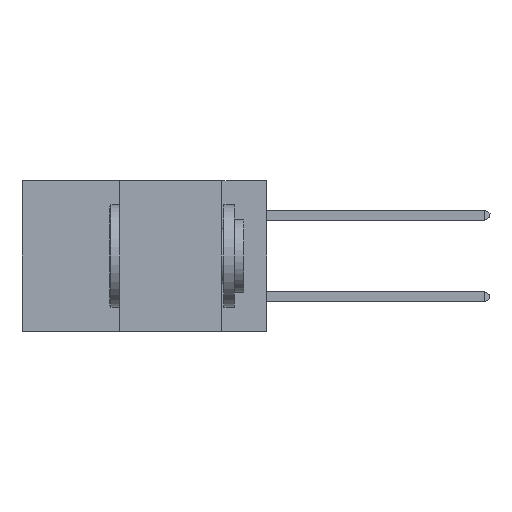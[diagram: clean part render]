
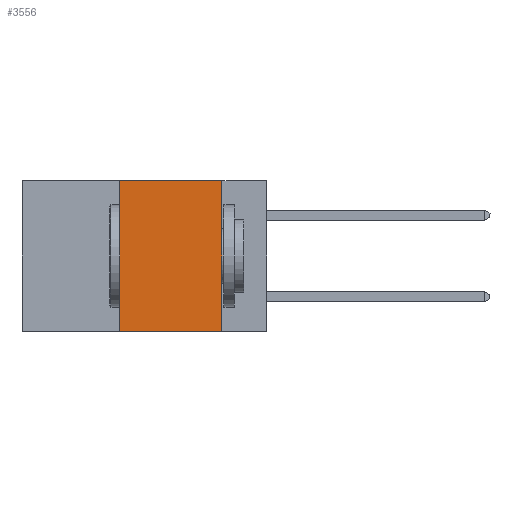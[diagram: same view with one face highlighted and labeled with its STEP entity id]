
A CAD part, left-side view. The second image highlights one B-rep face of the part: STEP entity #3556.
In plain terms, the highlighted planar face has unit normal (-1, 0, 0).
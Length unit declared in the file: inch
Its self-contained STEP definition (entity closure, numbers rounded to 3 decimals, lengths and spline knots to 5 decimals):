
#459 = ORIENTED_EDGE ( 'NONE', *, *, #3895, .F. ) ;
#595 = ORIENTED_EDGE ( 'NONE', *, *, #4956, .T. ) ;
#1918 = ORIENTED_EDGE ( 'NONE', *, *, #4938, .F. ) ;
#2269 = PLANE ( 'NONE',  #5113 ) ;
#2464 = LINE ( 'NONE', #4227, #11960 ) ;
#2852 = EDGE_CURVE ( 'NONE', #9878, #10428, #4239, .T. ) ;
#3326 = DIRECTION ( 'NONE',  ( 1., 0., 0. ) ) ;
#3556 = ADVANCED_FACE ( 'NONE', ( #12714 ), #2269, .F. ) ;
#3814 = CARTESIAN_POINT ( 'NONE',  ( 0., 0.36, 0. ) ) ;
#3895 = EDGE_CURVE ( 'NONE', #4630, #9878, #10008, .T. ) ;
#4008 = CARTESIAN_POINT ( 'NONE',  ( 0., 0.11, 0. ) ) ;
#4227 = CARTESIAN_POINT ( 'NONE',  ( 0., 0.6, -0.37 ) ) ;
#4239 = LINE ( 'NONE', #4814, #7137 ) ;
#4528 = VECTOR ( 'NONE', #10963, 39.37008 ) ;
#4630 = VERTEX_POINT ( 'NONE', #8724 ) ;
#4743 = DIRECTION ( 'NONE',  ( 0., -1., 0. ) ) ;
#4814 = CARTESIAN_POINT ( 'NONE',  ( 0., 0.6, 0. ) ) ;
#4938 = EDGE_CURVE ( 'NONE', #10428, #6269, #12277, .T. ) ;
#4956 = EDGE_CURVE ( 'NONE', #4630, #6269, #2464, .T. ) ;
#5113 = AXIS2_PLACEMENT_3D ( 'NONE', #9179, #3326, #10142 ) ;
#6191 = CARTESIAN_POINT ( 'NONE',  ( 0., 0.36, 0. ) ) ;
#6269 = VERTEX_POINT ( 'NONE', #7195 ) ;
#7137 = VECTOR ( 'NONE', #4743, 39.37008 ) ;
#7139 = EDGE_LOOP ( 'NONE', ( #1918, #9826, #459, #595 ) ) ;
#7195 = CARTESIAN_POINT ( 'NONE',  ( 0., 0.11, -0.37 ) ) ;
#7747 = VECTOR ( 'NONE', #11574, 39.37008 ) ;
#8724 = CARTESIAN_POINT ( 'NONE',  ( 0., 0.36, -0.37 ) ) ;
#9056 = CARTESIAN_POINT ( 'NONE',  ( 0., 0.11, 0. ) ) ;
#9179 = CARTESIAN_POINT ( 'NONE',  ( 0., 0.6, 0. ) ) ;
#9826 = ORIENTED_EDGE ( 'NONE', *, *, #2852, .F. ) ;
#9878 = VERTEX_POINT ( 'NONE', #6191 ) ;
#10008 = LINE ( 'NONE', #3814, #7747 ) ;
#10028 = DIRECTION ( 'NONE',  ( 0., -1., 0. ) ) ;
#10142 = DIRECTION ( 'NONE',  ( 0., 0., -1. ) ) ;
#10428 = VERTEX_POINT ( 'NONE', #4008 ) ;
#10963 = DIRECTION ( 'NONE',  ( 0., 0., -1. ) ) ;
#11574 = DIRECTION ( 'NONE',  ( 0., 0., 1. ) ) ;
#11960 = VECTOR ( 'NONE', #10028, 39.37008 ) ;
#12277 = LINE ( 'NONE', #9056, #4528 ) ;
#12714 = FACE_OUTER_BOUND ( 'NONE', #7139, .T. ) ;
